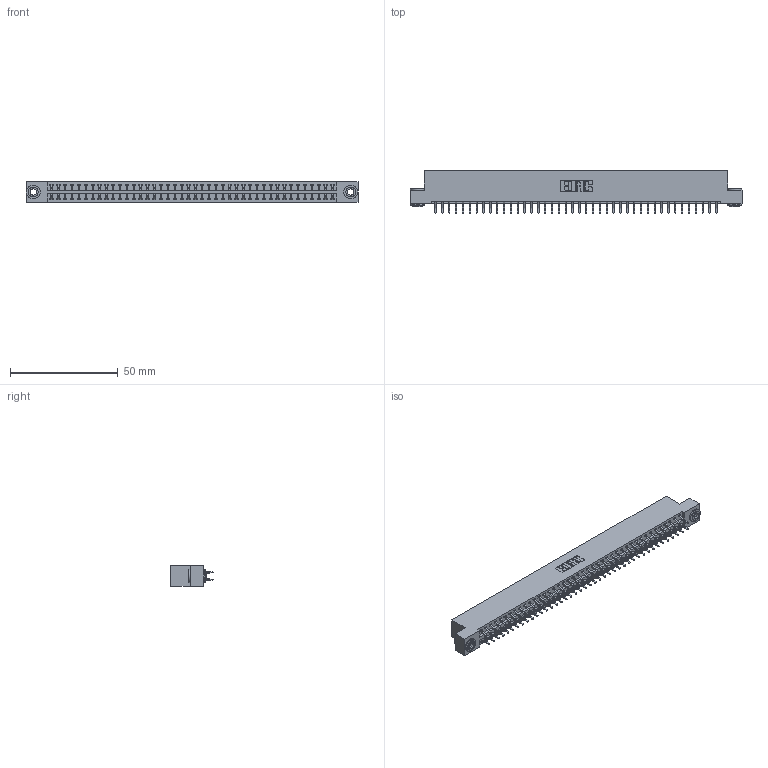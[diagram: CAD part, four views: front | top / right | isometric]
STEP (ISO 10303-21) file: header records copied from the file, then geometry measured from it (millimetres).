
FILE_DESCRIPTION (( 'STEP AP203' ), '1' );
FILE_NAME ('396-084-556-203.STEP', '2018-09-10T01:36:52', ( '' ), ( '' ), 'SwSTEP 2.0', 'SolidWorks 2016', '' );
FILE_SCHEMA (( 'CONFIG_CONTROL_DESIGN' ));
Length unit declared in the file: inch
Products named in the file (4): 346 Part_Flush Mounting Lugs - 0.156 Dia-TH; 345-292-001_556 Tail; 345-250-002_345-250-002-102; 396-084-556-203
Assembly tree (87 placements, depth 2):
  396-084-556-203
    346 Part_Flush Mounting Lugs - 0.156 Dia-TH
    345-292-001_556 Tail  x84
    345-250-002_345-250-002-102  x2
Bounding box: 153.92 x 19.57 x 9.4 mm (x, y, z)
Volume: 15025.6 mm3; surface area: 20789.8 mm2
Topology: 87 solids, 87 shells, 5032 faces, 14937 edges, 9842 vertices
Faces by surface type: plane 3362, cylinder 1662, cone 8
Entity records: 28280 total; most frequent: CARTESIAN_POINT 4651, ORIENTED_EDGE 4566, DIRECTION 4169, EDGE_CURVE 2283, LINE 1951, VECTOR 1951, VERTEX_POINT 1518, AXIS2_PLACEMENT_3D 1109
